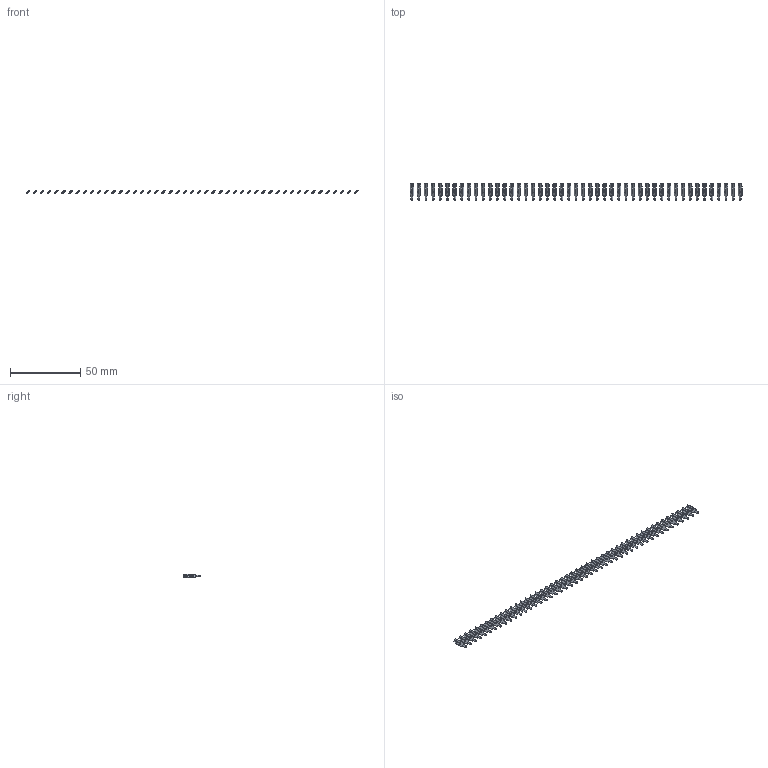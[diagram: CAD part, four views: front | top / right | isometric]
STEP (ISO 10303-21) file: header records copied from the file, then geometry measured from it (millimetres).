
FILE_DESCRIPTION (( 'STEP AP203' ), '1' );
FILE_NAME ('106-047-250-200.STEP', '2020-04-16T20:26:03', ( '' ), ( '' ), 'SwSTEP 2.0', 'SolidWorks 2016', '' );
FILE_SCHEMA (( 'CONFIG_CONTROL_DESIGN' ));
Length unit declared in the file: inch
Products named in the file (2): 100-290-001_100-290-250; 106-047-250-200
Assembly tree (47 placements, depth 2):
  106-047-250-200
    100-290-001_100-290-250  x47
Bounding box: 236.21 x 11.48 x 2.53 mm (x, y, z)
Volume: 733.4 mm3; surface area: 3447.4 mm2
Topology: 47 solids, 47 shells, 1128 faces, 3102 edges, 2068 vertices
Faces by surface type: plane 940, cylinder 188
Entity records: 2430 total; most frequent: DIRECTION 218, CARTESIAN_POINT 196, ORIENTED_EDGE 132, COORDINATED_UNIVERSAL_TIME_OFFSET 104, CALENDAR_DATE 104, DATE_AND_TIME 104, LOCAL_TIME 104, AXIS2_PLACEMENT_3D 82
